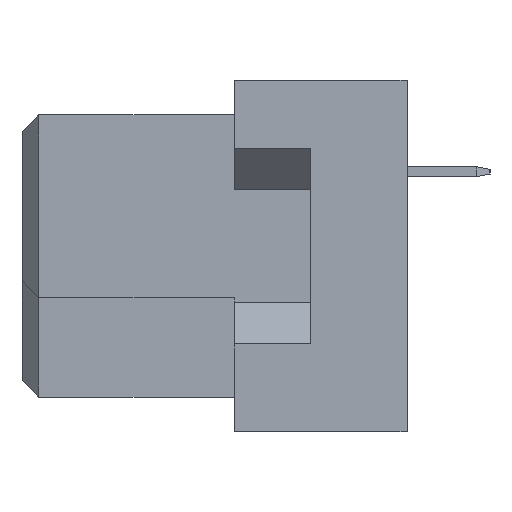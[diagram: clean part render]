
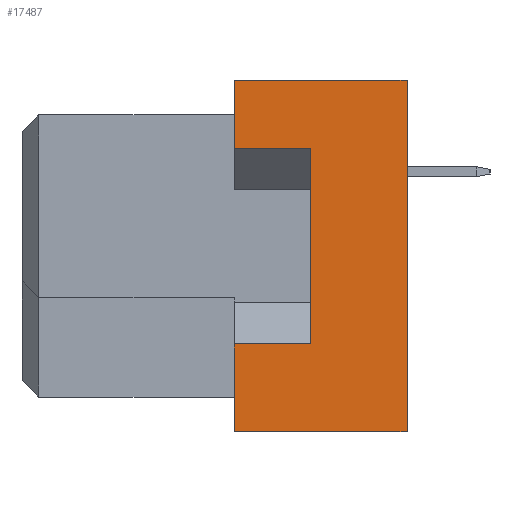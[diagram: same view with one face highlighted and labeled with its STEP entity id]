
A CAD part, left-side view. The second image highlights one B-rep face of the part: STEP entity #17487.
In plain terms, the highlighted planar face has unit normal (-1, 0, 0).
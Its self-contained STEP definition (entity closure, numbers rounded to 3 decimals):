
#120 = CARTESIAN_POINT ( 'NONE',  ( -27.5, -11.6, 5.3 ) ) ;
#692 = VECTOR ( 'NONE', #11862, 1000. ) ;
#831 = VECTOR ( 'NONE', #18985, 1000. ) ;
#2643 = LINE ( 'NONE', #13506, #692 ) ;
#2734 = EDGE_CURVE ( 'NONE', #3266, #15811, #7384, .T. ) ;
#2814 = VECTOR ( 'NONE', #5316, 1000. ) ;
#3266 = VERTEX_POINT ( 'NONE', #12309 ) ;
#3911 = CARTESIAN_POINT ( 'NONE',  ( -27.5, -8.7, 3.25 ) ) ;
#4517 = CARTESIAN_POINT ( 'NONE',  ( -27.5, -6.4, 5.3 ) ) ;
#5134 = LINE ( 'NONE', #6774, #14932 ) ;
#5146 = EDGE_CURVE ( 'NONE', #12108, #15811, #2643, .T. ) ;
#5316 = DIRECTION ( 'NONE',  ( 0., 0., 1. ) ) ;
#5452 = VECTOR ( 'NONE', #8606, 1000. ) ;
#5639 = LINE ( 'NONE', #18361, #14400 ) ;
#5655 = DIRECTION ( 'NONE',  ( 0., 1., 0. ) ) ;
#6013 = EDGE_CURVE ( 'NONE', #3266, #7399, #5639, .T. ) ;
#6049 = ORIENTED_EDGE ( 'NONE', *, *, #7780, .T. ) ;
#6093 = DIRECTION ( 'NONE',  ( 0., 0., 1. ) ) ;
#6619 = CARTESIAN_POINT ( 'NONE',  ( -27.5, -11.6, -5.3 ) ) ;
#6774 = CARTESIAN_POINT ( 'NONE',  ( -27.5, -6.4, -5.3 ) ) ;
#7004 = ORIENTED_EDGE ( 'NONE', *, *, #8393, .T. ) ;
#7161 = ORIENTED_EDGE ( 'NONE', *, *, #2734, .T. ) ;
#7173 = DIRECTION ( 'NONE',  ( 0., 0., 1. ) ) ;
#7384 = LINE ( 'NONE', #13647, #18628 ) ;
#7399 = VERTEX_POINT ( 'NONE', #12369 ) ;
#7780 = EDGE_CURVE ( 'NONE', #13940, #11859, #7901, .T. ) ;
#7901 = LINE ( 'NONE', #120, #831 ) ;
#8393 = EDGE_CURVE ( 'NONE', #8756, #13940, #14522, .T. ) ;
#8606 = DIRECTION ( 'NONE',  ( 0., 1., 0. ) ) ;
#8756 = VERTEX_POINT ( 'NONE', #6619 ) ;
#8964 = FACE_OUTER_BOUND ( 'NONE', #15417, .T. ) ;
#9545 = VECTOR ( 'NONE', #19756, 1000. ) ;
#10114 = ORIENTED_EDGE ( 'NONE', *, *, #15919, .F. ) ;
#10192 = ORIENTED_EDGE ( 'NONE', *, *, #18315, .F. ) ;
#10687 = ORIENTED_EDGE ( 'NONE', *, *, #5146, .F. ) ;
#10715 = CARTESIAN_POINT ( 'NONE',  ( -27.5, -11.6, 5.3 ) ) ;
#10987 = CARTESIAN_POINT ( 'NONE',  ( -27.5, -11.6, 5.3 ) ) ;
#11388 = DIRECTION ( 'NONE',  ( 0., 0., 1. ) ) ;
#11859 = VERTEX_POINT ( 'NONE', #4517 ) ;
#11862 = DIRECTION ( 'NONE',  ( 0., 0., 1. ) ) ;
#11863 = CARTESIAN_POINT ( 'NONE',  ( -27.5, -11.6, -5.3 ) ) ;
#11884 = ORIENTED_EDGE ( 'NONE', *, *, #18584, .F. ) ;
#12108 = VERTEX_POINT ( 'NONE', #18515 ) ;
#12242 = DIRECTION ( 'NONE',  ( -1., 0., 0. ) ) ;
#12309 = CARTESIAN_POINT ( 'NONE',  ( -27.5, -8.7, -2.65 ) ) ;
#12369 = CARTESIAN_POINT ( 'NONE',  ( -27.5, -8.7, 3.25 ) ) ;
#12788 = CARTESIAN_POINT ( 'NONE',  ( -27.5, -6.4, 3.25 ) ) ;
#13506 = CARTESIAN_POINT ( 'NONE',  ( -27.5, -6.4, -5.3 ) ) ;
#13647 = CARTESIAN_POINT ( 'NONE',  ( -27.5, -8.7, -2.65 ) ) ;
#13871 = PLANE ( 'NONE',  #14897 ) ;
#13891 = LINE ( 'NONE', #11863, #9545 ) ;
#13940 = VERTEX_POINT ( 'NONE', #10987 ) ;
#14097 = ORIENTED_EDGE ( 'NONE', *, *, #6013, .F. ) ;
#14400 = VECTOR ( 'NONE', #7173, 1000. ) ;
#14514 = CARTESIAN_POINT ( 'NONE',  ( -27.5, -6.4, -2.65 ) ) ;
#14522 = LINE ( 'NONE', #19362, #2814 ) ;
#14897 = AXIS2_PLACEMENT_3D ( 'NONE', #10715, #12242, #6093 ) ;
#14932 = VECTOR ( 'NONE', #11388, 1000. ) ;
#15417 = EDGE_LOOP ( 'NONE', ( #7161, #10687, #10114, #7004, #6049, #11884, #10192, #14097 ) ) ;
#15641 = VERTEX_POINT ( 'NONE', #12788 ) ;
#15811 = VERTEX_POINT ( 'NONE', #14514 ) ;
#15919 = EDGE_CURVE ( 'NONE', #8756, #12108, #13891, .T. ) ;
#16624 = LINE ( 'NONE', #3911, #5452 ) ;
#17487 = ADVANCED_FACE ( 'NONE', ( #8964 ), #13871, .T. ) ;
#18315 = EDGE_CURVE ( 'NONE', #7399, #15641, #16624, .T. ) ;
#18361 = CARTESIAN_POINT ( 'NONE',  ( -27.5, -8.7, -2.65 ) ) ;
#18515 = CARTESIAN_POINT ( 'NONE',  ( -27.5, -6.4, -5.3 ) ) ;
#18584 = EDGE_CURVE ( 'NONE', #15641, #11859, #5134, .T. ) ;
#18628 = VECTOR ( 'NONE', #5655, 1000. ) ;
#18985 = DIRECTION ( 'NONE',  ( 0., 1., 0. ) ) ;
#19362 = CARTESIAN_POINT ( 'NONE',  ( -27.5, -11.6, 5.3 ) ) ;
#19756 = DIRECTION ( 'NONE',  ( 0., 1., 0. ) ) ;
